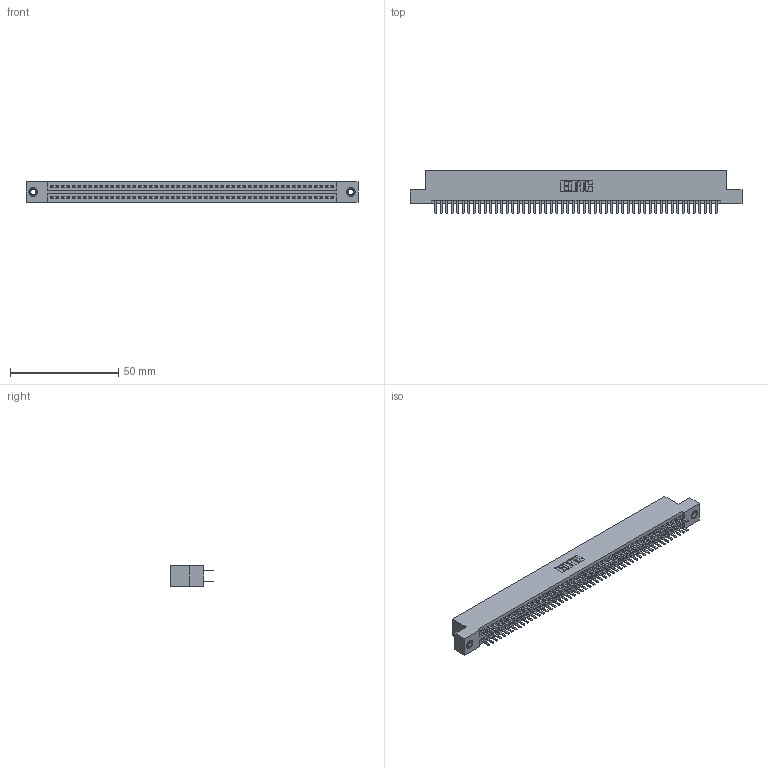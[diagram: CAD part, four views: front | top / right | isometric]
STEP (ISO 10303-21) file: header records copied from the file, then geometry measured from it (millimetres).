
FILE_DESCRIPTION (( 'STEP AP203' ), '1' );
FILE_NAME ('345-104-520-207.STEP', '2019-11-03T10:16:24', ( '' ), ( '' ), 'SwSTEP 2.0', 'SolidWorks 2016', '' );
FILE_SCHEMA (( 'CONFIG_CONTROL_DESIGN' ));
Length unit declared in the file: inch
Products named in the file (4): 345 Part_Flush Mounting Lugs - 0.156 Dia-TI; 345-292-001_345-293-120; 345-104-520-207; 345-250-001_345-250-005-103
Assembly tree (107 placements, depth 2):
  345-104-520-207
    345 Part_Flush Mounting Lugs - 0.156 Dia-TI
    345-292-001_345-293-120  x104
    345-250-001_345-250-005-103  x2
Bounding box: 153.29 x 19.68 x 9.4 mm (x, y, z)
Volume: 14924.2 mm3; surface area: 22184.8 mm2
Topology: 107 solids, 107 shells, 5802 faces, 16805 edges, 10918 vertices
Faces by surface type: plane 3752, cylinder 2034, cone 12, torus 4
Entity records: 40754 total; most frequent: CARTESIAN_POINT 6815, ORIENTED_EDGE 6730, DIRECTION 6011, EDGE_CURVE 3365, LINE 3001, VECTOR 3001, VERTEX_POINT 2236, AXIS2_PLACEMENT_3D 1505
